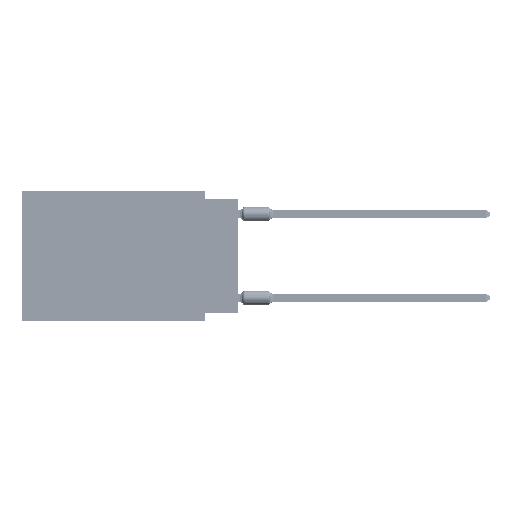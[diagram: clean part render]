
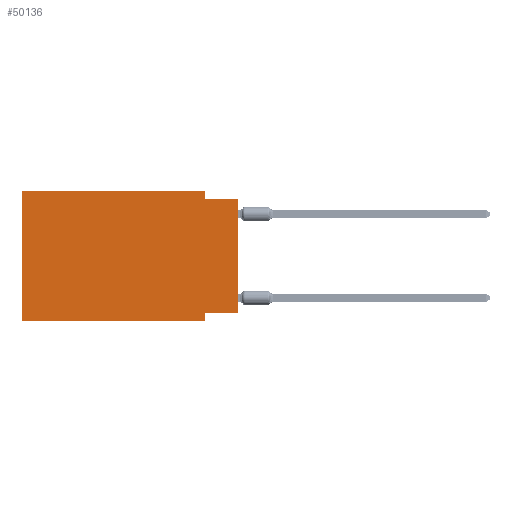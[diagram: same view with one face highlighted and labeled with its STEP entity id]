
A CAD part, left-side view. The second image highlights one B-rep face of the part: STEP entity #50136.
In plain terms, the highlighted planar face has unit normal (-1, 0, 0).
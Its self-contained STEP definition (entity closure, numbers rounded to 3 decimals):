
#2776 = LINE ( 'NONE', #32185, #15827 ) ;
#4183 = CARTESIAN_POINT ( 'NONE',  ( 0., 16.383, -9.906 ) ) ;
#4363 = ORIENTED_EDGE ( 'NONE', *, *, #72289, .F. ) ;
#5329 = LINE ( 'NONE', #46878, #7500 ) ;
#7057 = VECTOR ( 'NONE', #66280, 1000. ) ;
#7500 = VECTOR ( 'NONE', #35500, 1000. ) ;
#8024 = FACE_OUTER_BOUND ( 'NONE', #19605, .T. ) ;
#11707 = DIRECTION ( 'NONE',  ( 0., -1., 0. ) ) ;
#11967 = LINE ( 'NONE', #54698, #37678 ) ;
#13162 = CARTESIAN_POINT ( 'NONE',  ( 0., 16.383, 0. ) ) ;
#14741 = LINE ( 'NONE', #44142, #53239 ) ;
#15451 = CARTESIAN_POINT ( 'NONE',  ( 0., 16.383, 0. ) ) ;
#15827 = VECTOR ( 'NONE', #67859, 1000. ) ;
#17086 = EDGE_CURVE ( 'NONE', #71294, #49583, #41997, .T. ) ;
#17702 = ORIENTED_EDGE ( 'NONE', *, *, #36042, .F. ) ;
#19605 = EDGE_LOOP ( 'NONE', ( #27979, #44372, #71114, #51777, #4363, #24937, #59656, #17702 ) ) ;
#22777 = VECTOR ( 'NONE', #11707, 1000. ) ;
#22861 = CARTESIAN_POINT ( 'NONE',  ( 0., 16.383, -9.906 ) ) ;
#23254 = LINE ( 'NONE', #22861, #63630 ) ;
#24937 = ORIENTED_EDGE ( 'NONE', *, *, #68094, .T. ) ;
#27979 = ORIENTED_EDGE ( 'NONE', *, *, #71195, .T. ) ;
#28274 = VERTEX_POINT ( 'NONE', #13162 ) ;
#28735 = DIRECTION ( 'NONE',  ( 0., -1., 0. ) ) ;
#31190 = LINE ( 'NONE', #73856, #36972 ) ;
#31965 = DIRECTION ( 'NONE',  ( 0., 1., 0. ) ) ;
#32185 = CARTESIAN_POINT ( 'NONE',  ( 0., 2.54, 0. ) ) ;
#32684 = CARTESIAN_POINT ( 'NONE',  ( 0., 2.54, -9.271 ) ) ;
#34069 = AXIS2_PLACEMENT_3D ( 'NONE', #15451, #44837, #56628 ) ;
#35500 = DIRECTION ( 'NONE',  ( 0., 0., 1. ) ) ;
#36042 = EDGE_CURVE ( 'NONE', #44717, #71294, #31190, .T. ) ;
#36972 = VECTOR ( 'NONE', #31965, 1000. ) ;
#37145 = CARTESIAN_POINT ( 'NONE',  ( 0., 2.54, -9.906 ) ) ;
#37678 = VECTOR ( 'NONE', #60557, 1000. ) ;
#40906 = CARTESIAN_POINT ( 'NONE',  ( 0., 0., -9.271 ) ) ;
#41997 = LINE ( 'NONE', #54179, #7057 ) ;
#44142 = CARTESIAN_POINT ( 'NONE',  ( 0., 0., -0.635 ) ) ;
#44149 = VERTEX_POINT ( 'NONE', #57896 ) ;
#44372 = ORIENTED_EDGE ( 'NONE', *, *, #64178, .F. ) ;
#44717 = VERTEX_POINT ( 'NONE', #40906 ) ;
#44837 = DIRECTION ( 'NONE',  ( 1., 0., 0. ) ) ;
#45234 = PLANE ( 'NONE',  #34069 ) ;
#46878 = CARTESIAN_POINT ( 'NONE',  ( 0., 16.383, 0. ) ) ;
#49583 = VERTEX_POINT ( 'NONE', #37145 ) ;
#50136 = ADVANCED_FACE ( 'NONE', ( #8024 ), #45234, .F. ) ;
#50548 = EDGE_CURVE ( 'NONE', #28274, #60143, #71266, .T. ) ;
#51777 = ORIENTED_EDGE ( 'NONE', *, *, #50548, .F. ) ;
#53239 = VECTOR ( 'NONE', #72773, 1000. ) ;
#54179 = CARTESIAN_POINT ( 'NONE',  ( 0., 2.54, -9.906 ) ) ;
#54698 = CARTESIAN_POINT ( 'NONE',  ( 0., 0., 0. ) ) ;
#56628 = DIRECTION ( 'NONE',  ( 0., 0., -1. ) ) ;
#57896 = CARTESIAN_POINT ( 'NONE',  ( 0., 0., -0.635 ) ) ;
#58757 = CARTESIAN_POINT ( 'NONE',  ( 0., 16.383, 0. ) ) ;
#59178 = VERTEX_POINT ( 'NONE', #74397 ) ;
#59544 = VERTEX_POINT ( 'NONE', #4183 ) ;
#59656 = ORIENTED_EDGE ( 'NONE', *, *, #17086, .F. ) ;
#60143 = VERTEX_POINT ( 'NONE', #66643 ) ;
#60557 = DIRECTION ( 'NONE',  ( 0., 0., 1. ) ) ;
#63630 = VECTOR ( 'NONE', #28735, 1000. ) ;
#64178 = EDGE_CURVE ( 'NONE', #59178, #44149, #14741, .T. ) ;
#66280 = DIRECTION ( 'NONE',  ( 0., 0., -1. ) ) ;
#66643 = CARTESIAN_POINT ( 'NONE',  ( 0., 2.54, 0. ) ) ;
#67203 = EDGE_CURVE ( 'NONE', #60143, #59178, #2776, .T. ) ;
#67859 = DIRECTION ( 'NONE',  ( 0., 0., -1. ) ) ;
#68094 = EDGE_CURVE ( 'NONE', #59544, #49583, #23254, .T. ) ;
#71114 = ORIENTED_EDGE ( 'NONE', *, *, #67203, .F. ) ;
#71195 = EDGE_CURVE ( 'NONE', #44717, #44149, #11967, .T. ) ;
#71266 = LINE ( 'NONE', #58757, #22777 ) ;
#71294 = VERTEX_POINT ( 'NONE', #32684 ) ;
#72289 = EDGE_CURVE ( 'NONE', #59544, #28274, #5329, .T. ) ;
#72773 = DIRECTION ( 'NONE',  ( 0., -1., 0. ) ) ;
#73856 = CARTESIAN_POINT ( 'NONE',  ( 0., 0., -9.271 ) ) ;
#74397 = CARTESIAN_POINT ( 'NONE',  ( 0., 2.54, -0.635 ) ) ;
